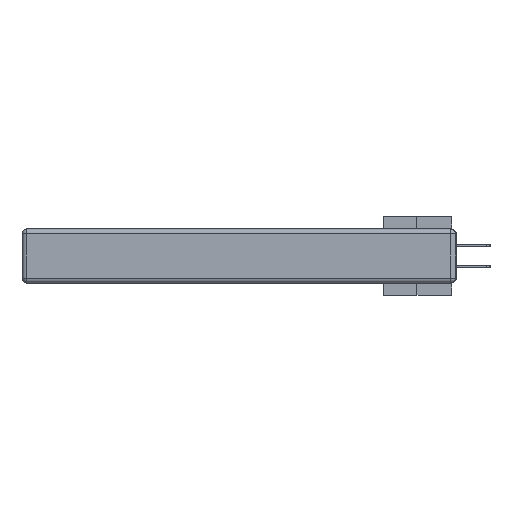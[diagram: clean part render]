
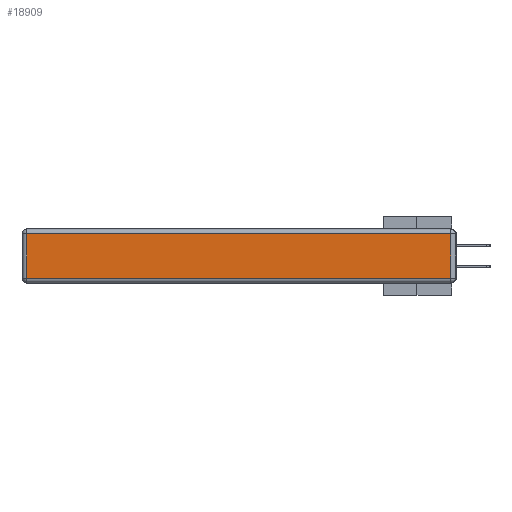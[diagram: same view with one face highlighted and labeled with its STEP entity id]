
A CAD part, left-side view. The second image highlights one B-rep face of the part: STEP entity #18909.
In plain terms, the highlighted planar face has unit normal (-1, 0, 0).
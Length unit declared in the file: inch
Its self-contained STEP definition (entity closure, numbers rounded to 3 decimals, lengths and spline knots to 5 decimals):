
#87 = DIRECTION ( 'NONE',  ( 0., -1., 0. ) ) ;
#416 = VERTEX_POINT ( 'NONE', #26285 ) ;
#2234 = EDGE_CURVE ( 'NONE', #5864, #22311, #20758, .T. ) ;
#2328 = CARTESIAN_POINT ( 'NONE',  ( 0., 2.72, -0.03 ) ) ;
#3222 = LINE ( 'NONE', #37375, #17364 ) ;
#3346 = ORIENTED_EDGE ( 'NONE', *, *, #18577, .T. ) ;
#5864 = VERTEX_POINT ( 'NONE', #7954 ) ;
#7954 = CARTESIAN_POINT ( 'NONE',  ( 0., 0.03, -0.03 ) ) ;
#10812 = EDGE_CURVE ( 'NONE', #416, #5864, #19588, .T. ) ;
#11032 = EDGE_LOOP ( 'NONE', ( #3346, #28480, #23171, #34668 ) ) ;
#11035 = FACE_OUTER_BOUND ( 'NONE', #11032, .T. ) ;
#11156 = DIRECTION ( 'NONE',  ( -1., 0., 0. ) ) ;
#11418 = CARTESIAN_POINT ( 'NONE',  ( 0., 0., -0.343 ) ) ;
#14102 = CARTESIAN_POINT ( 'NONE',  ( 0., 2.75, -0.03 ) ) ;
#14219 = VECTOR ( 'NONE', #18038, 39.37008 ) ;
#17364 = VECTOR ( 'NONE', #87, 39.37008 ) ;
#18038 = DIRECTION ( 'NONE',  ( 0., 0., 1. ) ) ;
#18577 = EDGE_CURVE ( 'NONE', #30478, #416, #3222, .T. ) ;
#18909 = ADVANCED_FACE ( 'NONE', ( #11035 ), #23653, .T. ) ;
#19588 = LINE ( 'NONE', #33641, #14219 ) ;
#20758 = LINE ( 'NONE', #14102, #34989 ) ;
#22311 = VERTEX_POINT ( 'NONE', #2328 ) ;
#22770 = DIRECTION ( 'NONE',  ( 0., 0., -1. ) ) ;
#23171 = ORIENTED_EDGE ( 'NONE', *, *, #2234, .T. ) ;
#23653 = PLANE ( 'NONE',  #31562 ) ;
#26285 = CARTESIAN_POINT ( 'NONE',  ( 0., 0.03, -0.313 ) ) ;
#27279 = DIRECTION ( 'NONE',  ( 0., 1., 0. ) ) ;
#28480 = ORIENTED_EDGE ( 'NONE', *, *, #10812, .T. ) ;
#30478 = VERTEX_POINT ( 'NONE', #40346 ) ;
#31562 = AXIS2_PLACEMENT_3D ( 'NONE', #11418, #11156, #36377 ) ;
#31839 = LINE ( 'NONE', #35626, #39115 ) ;
#33641 = CARTESIAN_POINT ( 'NONE',  ( 0., 0.03, -0.343 ) ) ;
#34668 = ORIENTED_EDGE ( 'NONE', *, *, #36450, .T. ) ;
#34989 = VECTOR ( 'NONE', #27279, 39.37008 ) ;
#35626 = CARTESIAN_POINT ( 'NONE',  ( 0., 2.72, -0.343 ) ) ;
#36377 = DIRECTION ( 'NONE',  ( 0., 0., 1. ) ) ;
#36450 = EDGE_CURVE ( 'NONE', #22311, #30478, #31839, .T. ) ;
#37375 = CARTESIAN_POINT ( 'NONE',  ( 0., 0., -0.313 ) ) ;
#39115 = VECTOR ( 'NONE', #22770, 39.37008 ) ;
#40346 = CARTESIAN_POINT ( 'NONE',  ( 0., 2.72, -0.313 ) ) ;
